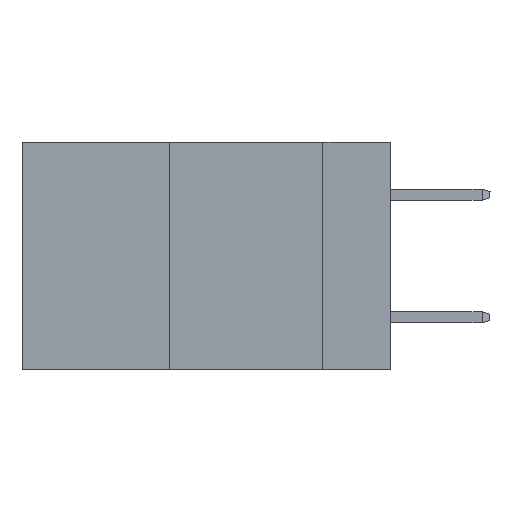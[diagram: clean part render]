
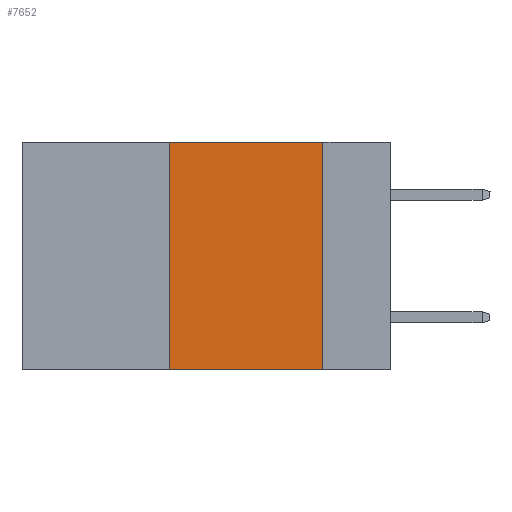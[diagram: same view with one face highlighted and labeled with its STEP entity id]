
A CAD part, left-side view. The second image highlights one B-rep face of the part: STEP entity #7652.
In plain terms, the highlighted planar face has unit normal (-1, 0, 0).
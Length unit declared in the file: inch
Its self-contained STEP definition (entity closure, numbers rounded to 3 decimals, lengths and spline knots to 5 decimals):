
#1123 = EDGE_CURVE ( 'NONE', #8634, #4243, #1967, .T. ) ;
#1525 = ORIENTED_EDGE ( 'NONE', *, *, #12742, .T. ) ;
#1967 = LINE ( 'NONE', #9334, #4653 ) ;
#2238 = VERTEX_POINT ( 'NONE', #5585 ) ;
#2384 = LINE ( 'NONE', #4626, #13712 ) ;
#2914 = CARTESIAN_POINT ( 'NONE',  ( 0., 0.36, 0. ) ) ;
#3946 = CARTESIAN_POINT ( 'NONE',  ( 0., 0.11, 0. ) ) ;
#4172 = DIRECTION ( 'NONE',  ( 0., 0., -1. ) ) ;
#4243 = VERTEX_POINT ( 'NONE', #3946 ) ;
#4626 = CARTESIAN_POINT ( 'NONE',  ( 0., 0.6, -0.37 ) ) ;
#4653 = VECTOR ( 'NONE', #7777, 39.37008 ) ;
#4738 = ORIENTED_EDGE ( 'NONE', *, *, #11050, .F. ) ;
#4937 = CARTESIAN_POINT ( 'NONE',  ( 0., 0.11, -0.37 ) ) ;
#5169 = DIRECTION ( 'NONE',  ( 0., 0., -1. ) ) ;
#5263 = FACE_OUTER_BOUND ( 'NONE', #7234, .T. ) ;
#5585 = CARTESIAN_POINT ( 'NONE',  ( 0., 0.36, -0.37 ) ) ;
#6774 = VECTOR ( 'NONE', #4172, 39.37008 ) ;
#7234 = EDGE_LOOP ( 'NONE', ( #4738, #13406, #11963, #1525 ) ) ;
#7652 = ADVANCED_FACE ( 'NONE', ( #5263 ), #12755, .F. ) ;
#7777 = DIRECTION ( 'NONE',  ( 0., -1., 0. ) ) ;
#7974 = LINE ( 'NONE', #2914, #10808 ) ;
#8153 = EDGE_CURVE ( 'NONE', #2238, #8634, #7974, .T. ) ;
#8588 = CARTESIAN_POINT ( 'NONE',  ( 0., 0.6, 0. ) ) ;
#8634 = VERTEX_POINT ( 'NONE', #13912 ) ;
#9334 = CARTESIAN_POINT ( 'NONE',  ( 0., 0.6, 0. ) ) ;
#9799 = CARTESIAN_POINT ( 'NONE',  ( 0., 0.11, 0. ) ) ;
#10671 = DIRECTION ( 'NONE',  ( 0., 0., 1. ) ) ;
#10808 = VECTOR ( 'NONE', #10671, 39.37008 ) ;
#11050 = EDGE_CURVE ( 'NONE', #4243, #13669, #12513, .T. ) ;
#11747 = DIRECTION ( 'NONE',  ( 1., 0., 0. ) ) ;
#11963 = ORIENTED_EDGE ( 'NONE', *, *, #8153, .F. ) ;
#12271 = DIRECTION ( 'NONE',  ( 0., -1., 0. ) ) ;
#12513 = LINE ( 'NONE', #9799, #6774 ) ;
#12742 = EDGE_CURVE ( 'NONE', #2238, #13669, #2384, .T. ) ;
#12755 = PLANE ( 'NONE',  #13911 ) ;
#13406 = ORIENTED_EDGE ( 'NONE', *, *, #1123, .F. ) ;
#13669 = VERTEX_POINT ( 'NONE', #4937 ) ;
#13712 = VECTOR ( 'NONE', #12271, 39.37008 ) ;
#13911 = AXIS2_PLACEMENT_3D ( 'NONE', #8588, #11747, #5169 ) ;
#13912 = CARTESIAN_POINT ( 'NONE',  ( 0., 0.36, 0. ) ) ;
